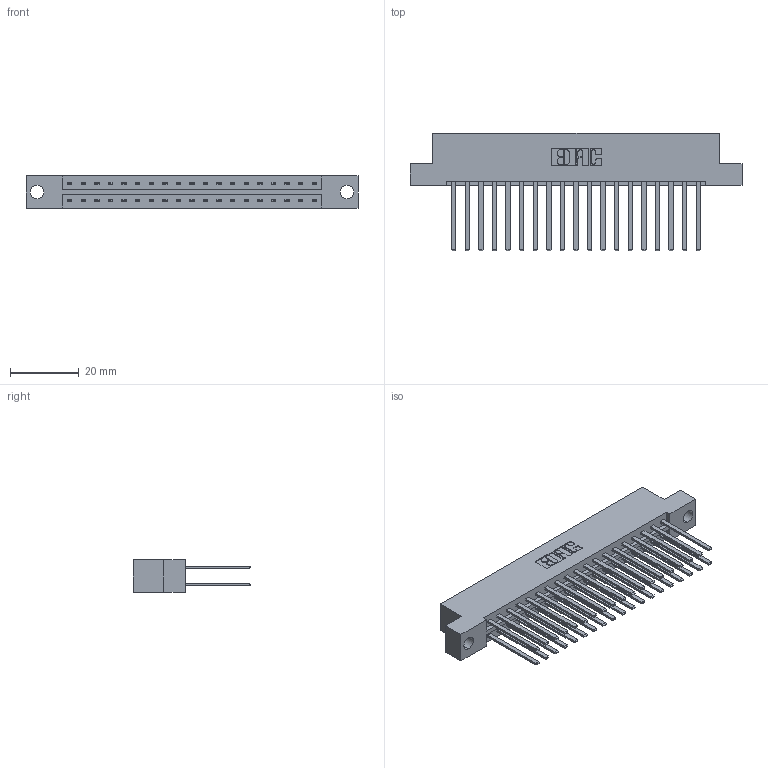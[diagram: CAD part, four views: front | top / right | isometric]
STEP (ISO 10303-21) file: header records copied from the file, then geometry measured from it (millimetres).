
FILE_DESCRIPTION (( 'STEP AP203' ), '1' );
FILE_NAME ('833-038-544-204.STEP', '2020-06-03T13:13:20', ( '' ), ( '' ), 'SwSTEP 2.0', 'SolidWorks 2020', '' );
FILE_SCHEMA (( 'CONFIG_CONTROL_DESIGN' ));
Length unit declared in the file: inch
Products named in the file (3): 833 Part_Flush - .156 Dia - TH; 345-292-001_345-293-144; 833-038-544-204
Assembly tree (39 placements, depth 2):
  833-038-544-204
    833 Part_Flush - .156 Dia - TH
    345-292-001_345-293-144  x38
Bounding box: 96.82 x 34.3 x 9.4 mm (x, y, z)
Volume: 10115 mm3; surface area: 13225.9 mm2
Topology: 39 solids, 39 shells, 1862 faces, 5517 edges, 3626 vertices
Faces by surface type: plane 1286, cylinder 576
Entity records: 15017 total; most frequent: CARTESIAN_POINT 2514, ORIENTED_EDGE 2450, DIRECTION 2185, EDGE_CURVE 1225, VECTOR 1101, LINE 1101, VERTEX_POINT 814, AXIS2_PLACEMENT_3D 542
